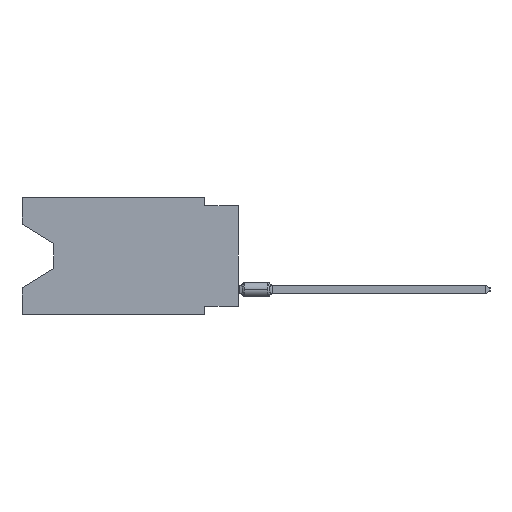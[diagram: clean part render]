
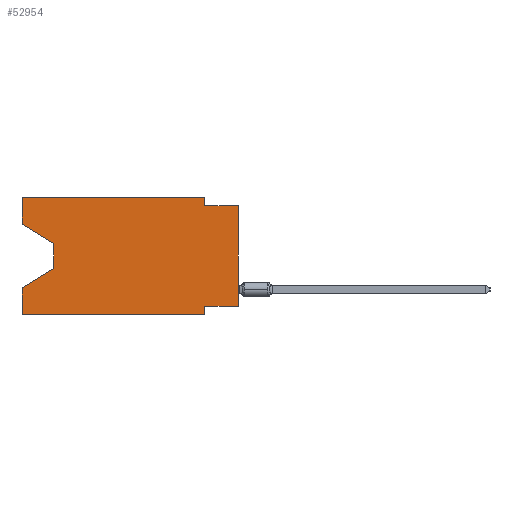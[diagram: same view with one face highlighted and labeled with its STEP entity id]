
A CAD part, left-side view. The second image highlights one B-rep face of the part: STEP entity #52954.
In plain terms, the highlighted planar face has unit normal (-1, 0, 0).
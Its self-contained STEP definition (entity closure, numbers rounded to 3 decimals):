
#184 = VECTOR ( 'NONE', #47863, 1000. ) ;
#1597 = CARTESIAN_POINT ( 'NONE',  ( 0., 16.383, 0. ) ) ;
#2958 = EDGE_CURVE ( 'NONE', #17025, #85762, #82052, .T. ) ;
#3315 = ORIENTED_EDGE ( 'NONE', *, *, #39137, .F. ) ;
#3523 = CARTESIAN_POINT ( 'NONE',  ( 0., 16.383, -6.852 ) ) ;
#4064 = CARTESIAN_POINT ( 'NONE',  ( 0., 0., -0.635 ) ) ;
#5067 = VECTOR ( 'NONE', #106319, 1000. ) ;
#6452 = CARTESIAN_POINT ( 'NONE',  ( 0., 13.97, -3.505 ) ) ;
#6473 = EDGE_CURVE ( 'NONE', #30014, #36465, #10278, .T. ) ;
#8176 = CARTESIAN_POINT ( 'NONE',  ( 0., 0., -0.635 ) ) ;
#8594 = DIRECTION ( 'NONE',  ( 0., -1., 0. ) ) ;
#8658 = VERTEX_POINT ( 'NONE', #69185 ) ;
#9247 = LINE ( 'NONE', #16832, #5067 ) ;
#10089 = CARTESIAN_POINT ( 'NONE',  ( 0., 2.54, 0. ) ) ;
#10278 = LINE ( 'NONE', #1597, #11900 ) ;
#11133 = CARTESIAN_POINT ( 'NONE',  ( 0., 0., 0. ) ) ;
#11667 = VERTEX_POINT ( 'NONE', #4064 ) ;
#11900 = VECTOR ( 'NONE', #68818, 1000. ) ;
#11913 = ORIENTED_EDGE ( 'NONE', *, *, #47233, .F. ) ;
#13071 = VECTOR ( 'NONE', #66308, 1000. ) ;
#13670 = DIRECTION ( 'NONE',  ( 0., 0., -1. ) ) ;
#15357 = ORIENTED_EDGE ( 'NONE', *, *, #83526, .F. ) ;
#16658 = CARTESIAN_POINT ( 'NONE',  ( 0., 13.97, -3.505 ) ) ;
#16832 = CARTESIAN_POINT ( 'NONE',  ( 0., 2.54, -8.89 ) ) ;
#17025 = VERTEX_POINT ( 'NONE', #59275 ) ;
#17929 = VECTOR ( 'NONE', #49834, 1000. ) ;
#18414 = ORIENTED_EDGE ( 'NONE', *, *, #106181, .T. ) ;
#19082 = VECTOR ( 'NONE', #62882, 1000. ) ;
#20223 = VECTOR ( 'NONE', #49165, 1000. ) ;
#21060 = VERTEX_POINT ( 'NONE', #105824 ) ;
#21068 = ORIENTED_EDGE ( 'NONE', *, *, #50565, .F. ) ;
#21810 = PLANE ( 'NONE',  #64572 ) ;
#22036 = EDGE_CURVE ( 'NONE', #99206, #21060, #27303, .T. ) ;
#23683 = LINE ( 'NONE', #81161, #20223 ) ;
#24894 = LINE ( 'NONE', #91044, #17929 ) ;
#25262 = LINE ( 'NONE', #11133, #98940 ) ;
#25693 = EDGE_LOOP ( 'NONE', ( #18414, #44244, #29765, #48777, #59684, #11913, #83754, #46956, #3315, #69739, #21068, #15357 ) ) ;
#27303 = LINE ( 'NONE', #50633, #74516 ) ;
#29765 = ORIENTED_EDGE ( 'NONE', *, *, #79817, .T. ) ;
#30014 = VERTEX_POINT ( 'NONE', #31828 ) ;
#30562 = CARTESIAN_POINT ( 'NONE',  ( 0., 13.97, -5.385 ) ) ;
#31828 = CARTESIAN_POINT ( 'NONE',  ( 0., 16.383, -8.89 ) ) ;
#32697 = CARTESIAN_POINT ( 'NONE',  ( 0., 0., -8.255 ) ) ;
#34186 = DIRECTION ( 'NONE',  ( 0., -1., 0. ) ) ;
#34358 = DIRECTION ( 'NONE',  ( 0., 0., -1. ) ) ;
#35470 = VERTEX_POINT ( 'NONE', #66857 ) ;
#36465 = VERTEX_POINT ( 'NONE', #3523 ) ;
#36563 = VECTOR ( 'NONE', #8594, 1000. ) ;
#39137 = EDGE_CURVE ( 'NONE', #21060, #11667, #75921, .T. ) ;
#40887 = VECTOR ( 'NONE', #34186, 1000. ) ;
#44244 = ORIENTED_EDGE ( 'NONE', *, *, #49956, .T. ) ;
#46956 = ORIENTED_EDGE ( 'NONE', *, *, #51077, .T. ) ;
#47233 = EDGE_CURVE ( 'NONE', #85762, #96035, #9247, .T. ) ;
#47863 = DIRECTION ( 'NONE',  ( 0., -0.855, -0.519 ) ) ;
#48400 = LINE ( 'NONE', #105877, #184 ) ;
#48777 = ORIENTED_EDGE ( 'NONE', *, *, #6473, .F. ) ;
#49165 = DIRECTION ( 'NONE',  ( 0., 0., 1. ) ) ;
#49834 = DIRECTION ( 'NONE',  ( 0., -1., 0. ) ) ;
#49956 = EDGE_CURVE ( 'NONE', #70519, #64889, #88888, .T. ) ;
#50565 = EDGE_CURVE ( 'NONE', #8658, #99206, #58442, .T. ) ;
#50633 = CARTESIAN_POINT ( 'NONE',  ( 0., 2.54, 0. ) ) ;
#51077 = EDGE_CURVE ( 'NONE', #17025, #11667, #25262, .T. ) ;
#52954 = ADVANCED_FACE ( 'NONE', ( #96094 ), #21810, .F. ) ;
#54894 = DIRECTION ( 'NONE',  ( 1., 0., 0. ) ) ;
#57912 = CARTESIAN_POINT ( 'NONE',  ( 0., 16.383, 0. ) ) ;
#58442 = LINE ( 'NONE', #57912, #36563 ) ;
#59275 = CARTESIAN_POINT ( 'NONE',  ( 0., 0., -8.255 ) ) ;
#59684 = ORIENTED_EDGE ( 'NONE', *, *, #73574, .T. ) ;
#62882 = DIRECTION ( 'NONE',  ( 0., 0., -1. ) ) ;
#64089 = CARTESIAN_POINT ( 'NONE',  ( 0., 16.383, 0. ) ) ;
#64572 = AXIS2_PLACEMENT_3D ( 'NONE', #64089, #54894, #13670 ) ;
#64889 = VERTEX_POINT ( 'NONE', #30562 ) ;
#66308 = DIRECTION ( 'NONE',  ( 0., 1., 0. ) ) ;
#66857 = CARTESIAN_POINT ( 'NONE',  ( 0., 16.383, -2.038 ) ) ;
#68818 = DIRECTION ( 'NONE',  ( 0., 0., 1. ) ) ;
#69185 = CARTESIAN_POINT ( 'NONE',  ( 0., 16.383, 0. ) ) ;
#69739 = ORIENTED_EDGE ( 'NONE', *, *, #22036, .F. ) ;
#70465 = CARTESIAN_POINT ( 'NONE',  ( 0., 2.54, -8.255 ) ) ;
#70519 = VERTEX_POINT ( 'NONE', #16658 ) ;
#73574 = EDGE_CURVE ( 'NONE', #30014, #96035, #24894, .T. ) ;
#74430 = DIRECTION ( 'NONE',  ( 0., 0.855, -0.519 ) ) ;
#74516 = VECTOR ( 'NONE', #34358, 1000. ) ;
#75921 = LINE ( 'NONE', #8176, #40887 ) ;
#79358 = CARTESIAN_POINT ( 'NONE',  ( 0., 2.54, -8.89 ) ) ;
#79817 = EDGE_CURVE ( 'NONE', #64889, #36465, #82040, .T. ) ;
#81161 = CARTESIAN_POINT ( 'NONE',  ( 0., 16.383, 0. ) ) ;
#82040 = LINE ( 'NONE', #100433, #85377 ) ;
#82052 = LINE ( 'NONE', #32697, #13071 ) ;
#83526 = EDGE_CURVE ( 'NONE', #35470, #8658, #23683, .T. ) ;
#83754 = ORIENTED_EDGE ( 'NONE', *, *, #2958, .F. ) ;
#85377 = VECTOR ( 'NONE', #74430, 1000. ) ;
#85762 = VERTEX_POINT ( 'NONE', #70465 ) ;
#86485 = DIRECTION ( 'NONE',  ( 0., 0., 1. ) ) ;
#88888 = LINE ( 'NONE', #6452, #19082 ) ;
#91044 = CARTESIAN_POINT ( 'NONE',  ( 0., 16.383, -8.89 ) ) ;
#96035 = VERTEX_POINT ( 'NONE', #79358 ) ;
#96094 = FACE_OUTER_BOUND ( 'NONE', #25693, .T. ) ;
#98940 = VECTOR ( 'NONE', #86485, 1000. ) ;
#99206 = VERTEX_POINT ( 'NONE', #10089 ) ;
#100433 = CARTESIAN_POINT ( 'NONE',  ( 0., 13.97, -5.385 ) ) ;
#105824 = CARTESIAN_POINT ( 'NONE',  ( 0., 2.54, -0.635 ) ) ;
#105877 = CARTESIAN_POINT ( 'NONE',  ( 0., 16.383, -2.038 ) ) ;
#106181 = EDGE_CURVE ( 'NONE', #35470, #70519, #48400, .T. ) ;
#106319 = DIRECTION ( 'NONE',  ( 0., 0., -1. ) ) ;
